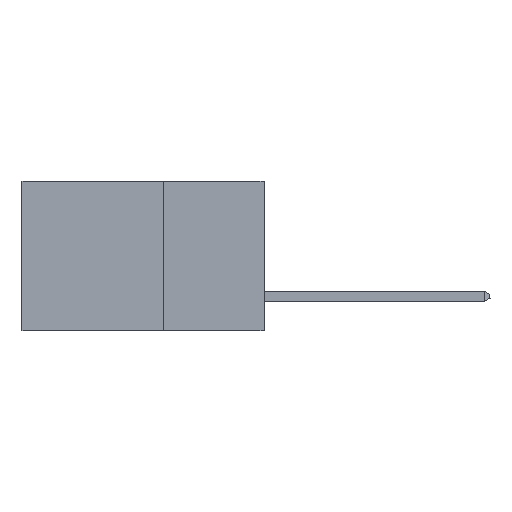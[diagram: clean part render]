
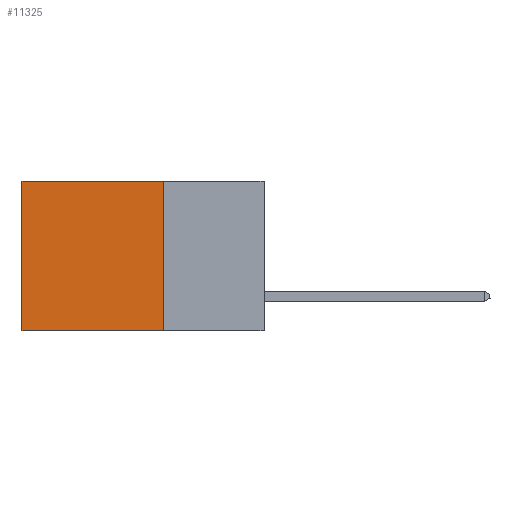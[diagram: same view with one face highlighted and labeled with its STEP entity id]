
A CAD part, left-side view. The second image highlights one B-rep face of the part: STEP entity #11325.
In plain terms, the highlighted planar face has unit normal (-1, 0, 0).
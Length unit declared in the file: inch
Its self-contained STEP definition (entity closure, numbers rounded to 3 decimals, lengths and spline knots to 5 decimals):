
#153 = VERTEX_POINT ( 'NONE', #9847 ) ;
#652 = CARTESIAN_POINT ( 'NONE',  ( 0.2615, 0.25, -0.37 ) ) ;
#2175 = LINE ( 'NONE', #12164, #4718 ) ;
#2221 = CARTESIAN_POINT ( 'NONE',  ( 0.2615, 0.25, -0.37 ) ) ;
#2490 = EDGE_CURVE ( 'NONE', #8287, #8234, #12105, .T. ) ;
#2950 = ORIENTED_EDGE ( 'NONE', *, *, #13985, .T. ) ;
#3144 = ORIENTED_EDGE ( 'NONE', *, *, #12580, .F. ) ;
#3164 = FACE_OUTER_BOUND ( 'NONE', #7829, .T. ) ;
#4497 = AXIS2_PLACEMENT_3D ( 'NONE', #13806, #5648, #9217 ) ;
#4601 = DIRECTION ( 'NONE',  ( 0., 1., 0. ) ) ;
#4718 = VECTOR ( 'NONE', #5311, 39.37008 ) ;
#5020 = CARTESIAN_POINT ( 'NONE',  ( 0.2615, 0.25, 0. ) ) ;
#5311 = DIRECTION ( 'NONE',  ( 0., 0., -1. ) ) ;
#5648 = DIRECTION ( 'NONE',  ( 1., 0., 0. ) ) ;
#5748 = ORIENTED_EDGE ( 'NONE', *, *, #2490, .T. ) ;
#5936 = CARTESIAN_POINT ( 'NONE',  ( 0.2615, 0.6, 0. ) ) ;
#7194 = EDGE_CURVE ( 'NONE', #8287, #13365, #2175, .T. ) ;
#7829 = EDGE_LOOP ( 'NONE', ( #2950, #3144, #10133, #5748 ) ) ;
#8234 = VERTEX_POINT ( 'NONE', #5936 ) ;
#8287 = VERTEX_POINT ( 'NONE', #8391 ) ;
#8391 = CARTESIAN_POINT ( 'NONE',  ( 0.2615, 0.25, 0. ) ) ;
#8456 = LINE ( 'NONE', #8664, #10778 ) ;
#8664 = CARTESIAN_POINT ( 'NONE',  ( 0.2615, 0.6, -0.37 ) ) ;
#9088 = VECTOR ( 'NONE', #9540, 39.37008 ) ;
#9217 = DIRECTION ( 'NONE',  ( 0., 0., -1. ) ) ;
#9540 = DIRECTION ( 'NONE',  ( 0., 1., 0. ) ) ;
#9847 = CARTESIAN_POINT ( 'NONE',  ( 0.2615, 0.6, -0.37 ) ) ;
#9873 = DIRECTION ( 'NONE',  ( 0., 0., -1. ) ) ;
#10133 = ORIENTED_EDGE ( 'NONE', *, *, #7194, .F. ) ;
#10293 = VECTOR ( 'NONE', #4601, 39.37008 ) ;
#10778 = VECTOR ( 'NONE', #9873, 39.37008 ) ;
#11325 = ADVANCED_FACE ( 'NONE', ( #3164 ), #12514, .F. ) ;
#12105 = LINE ( 'NONE', #5020, #9088 ) ;
#12164 = CARTESIAN_POINT ( 'NONE',  ( 0.2615, 0.25, -0.37 ) ) ;
#12514 = PLANE ( 'NONE',  #4497 ) ;
#12580 = EDGE_CURVE ( 'NONE', #13365, #153, #13141, .T. ) ;
#13141 = LINE ( 'NONE', #2221, #10293 ) ;
#13365 = VERTEX_POINT ( 'NONE', #652 ) ;
#13806 = CARTESIAN_POINT ( 'NONE',  ( 0.2615, 0.25, -0.37 ) ) ;
#13985 = EDGE_CURVE ( 'NONE', #8234, #153, #8456, .T. ) ;
